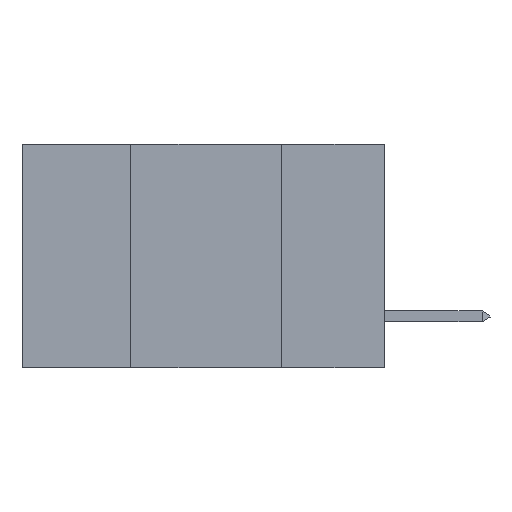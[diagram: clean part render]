
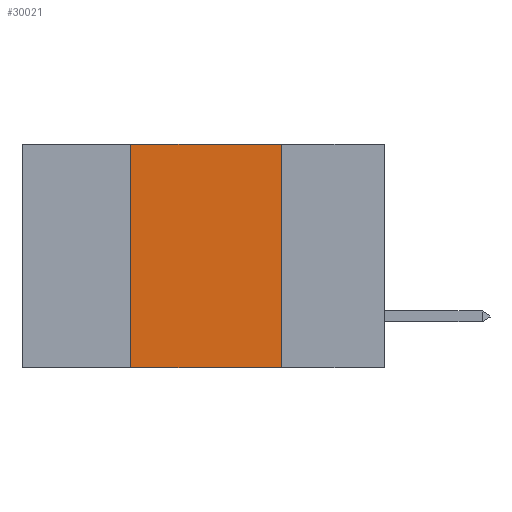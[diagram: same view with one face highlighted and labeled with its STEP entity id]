
A CAD part, left-side view. The second image highlights one B-rep face of the part: STEP entity #30021.
In plain terms, the highlighted planar face has unit normal (-1, 0, 0).
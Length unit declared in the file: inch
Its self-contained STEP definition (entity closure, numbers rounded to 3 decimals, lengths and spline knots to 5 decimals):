
#57 = LINE ( 'NONE', #4077, #26239 ) ;
#68 = LINE ( 'NONE', #11104, #12095 ) ;
#483 = ORIENTED_EDGE ( 'NONE', *, *, #36396, .F. ) ;
#1488 = EDGE_LOOP ( 'NONE', ( #26870, #483, #24566, #22007 ) ) ;
#4077 = CARTESIAN_POINT ( 'NONE',  ( 0., 0.6, -0.37 ) ) ;
#4148 = LINE ( 'NONE', #31407, #18428 ) ;
#5546 = VERTEX_POINT ( 'NONE', #7411 ) ;
#6974 = CARTESIAN_POINT ( 'NONE',  ( 0., 0.17, -0.37 ) ) ;
#7333 = EDGE_CURVE ( 'NONE', #30953, #16346, #32101, .T. ) ;
#7411 = CARTESIAN_POINT ( 'NONE',  ( 0., 0.17, 0. ) ) ;
#7511 = CARTESIAN_POINT ( 'NONE',  ( 0., 0.42, 0. ) ) ;
#8401 = EDGE_CURVE ( 'NONE', #30953, #31701, #57, .T. ) ;
#11104 = CARTESIAN_POINT ( 'NONE',  ( 0., 0.17, 0. ) ) ;
#11258 = VECTOR ( 'NONE', #27605, 39.37008 ) ;
#12095 = VECTOR ( 'NONE', #25468, 39.37008 ) ;
#14177 = DIRECTION ( 'NONE',  ( 0., -1., 0. ) ) ;
#15080 = FACE_OUTER_BOUND ( 'NONE', #1488, .T. ) ;
#16128 = CARTESIAN_POINT ( 'NONE',  ( 0., 0.6, 0. ) ) ;
#16250 = PLANE ( 'NONE',  #31926 ) ;
#16346 = VERTEX_POINT ( 'NONE', #25544 ) ;
#18428 = VECTOR ( 'NONE', #14177, 39.37008 ) ;
#20721 = CARTESIAN_POINT ( 'NONE',  ( 0., 0.42, -0.37 ) ) ;
#21822 = EDGE_CURVE ( 'NONE', #5546, #31701, #68, .T. ) ;
#22007 = ORIENTED_EDGE ( 'NONE', *, *, #8401, .T. ) ;
#22793 = DIRECTION ( 'NONE',  ( 1., 0., 0. ) ) ;
#24566 = ORIENTED_EDGE ( 'NONE', *, *, #7333, .F. ) ;
#25468 = DIRECTION ( 'NONE',  ( 0., 0., -1. ) ) ;
#25544 = CARTESIAN_POINT ( 'NONE',  ( 0., 0.42, 0. ) ) ;
#26239 = VECTOR ( 'NONE', #27287, 39.37008 ) ;
#26870 = ORIENTED_EDGE ( 'NONE', *, *, #21822, .F. ) ;
#27287 = DIRECTION ( 'NONE',  ( 0., -1., 0. ) ) ;
#27605 = DIRECTION ( 'NONE',  ( 0., 0., 1. ) ) ;
#30021 = ADVANCED_FACE ( 'NONE', ( #15080 ), #16250, .F. ) ;
#30953 = VERTEX_POINT ( 'NONE', #20721 ) ;
#30987 = DIRECTION ( 'NONE',  ( 0., 0., -1. ) ) ;
#31407 = CARTESIAN_POINT ( 'NONE',  ( 0., 0.6, 0. ) ) ;
#31701 = VERTEX_POINT ( 'NONE', #6974 ) ;
#31926 = AXIS2_PLACEMENT_3D ( 'NONE', #16128, #22793, #30987 ) ;
#32101 = LINE ( 'NONE', #7511, #11258 ) ;
#36396 = EDGE_CURVE ( 'NONE', #16346, #5546, #4148, .T. ) ;
